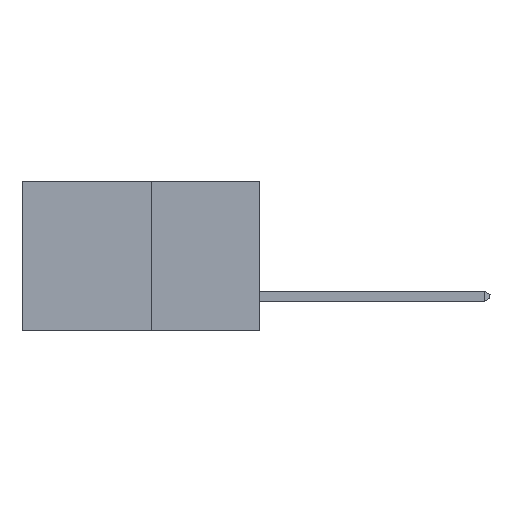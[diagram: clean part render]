
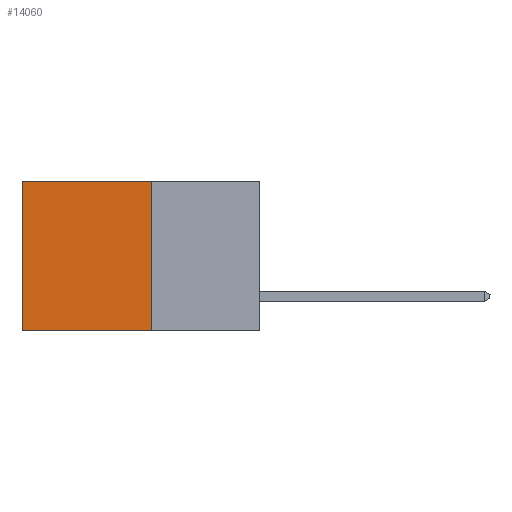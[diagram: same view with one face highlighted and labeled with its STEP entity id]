
A CAD part, left-side view. The second image highlights one B-rep face of the part: STEP entity #14060.
In plain terms, the highlighted planar face has unit normal (-1, 0, 0).
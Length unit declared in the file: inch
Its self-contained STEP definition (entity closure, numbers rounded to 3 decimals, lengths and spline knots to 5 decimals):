
#373 = CARTESIAN_POINT ( 'NONE',  ( 0.277, 0.59, -0.37 ) ) ;
#1002 = PLANE ( 'NONE',  #4621 ) ;
#1065 = EDGE_CURVE ( 'NONE', #9850, #3376, #4138, .T. ) ;
#1388 = VECTOR ( 'NONE', #14467, 39.37008 ) ;
#1573 = DIRECTION ( 'NONE',  ( 0., 0., -1. ) ) ;
#2392 = EDGE_LOOP ( 'NONE', ( #8125, #9862, #10087, #10769 ) ) ;
#2715 = CARTESIAN_POINT ( 'NONE',  ( 0.277, 0.27, -0.37 ) ) ;
#3339 = VECTOR ( 'NONE', #8155, 39.37008 ) ;
#3376 = VERTEX_POINT ( 'NONE', #4546 ) ;
#4138 = LINE ( 'NONE', #4902, #9516 ) ;
#4175 = LINE ( 'NONE', #6964, #1388 ) ;
#4546 = CARTESIAN_POINT ( 'NONE',  ( 0.277, 0.59, -0.37 ) ) ;
#4586 = DIRECTION ( 'NONE',  ( 1., 0., 0. ) ) ;
#4621 = AXIS2_PLACEMENT_3D ( 'NONE', #5686, #4586, #12361 ) ;
#4902 = CARTESIAN_POINT ( 'NONE',  ( 0.277, 0.27, -0.37 ) ) ;
#5686 = CARTESIAN_POINT ( 'NONE',  ( 0.277, 0.27, -0.37 ) ) ;
#5804 = CARTESIAN_POINT ( 'NONE',  ( 0.277, 0.59, 0. ) ) ;
#6320 = LINE ( 'NONE', #373, #9744 ) ;
#6578 = DIRECTION ( 'NONE',  ( 0., 1., 0. ) ) ;
#6732 = CARTESIAN_POINT ( 'NONE',  ( 0.277, 0.27, 0. ) ) ;
#6964 = CARTESIAN_POINT ( 'NONE',  ( 0.277, 0.27, -0.37 ) ) ;
#7525 = EDGE_CURVE ( 'NONE', #10479, #10148, #12274, .T. ) ;
#8125 = ORIENTED_EDGE ( 'NONE', *, *, #14337, .T. ) ;
#8155 = DIRECTION ( 'NONE',  ( 0., 1., 0. ) ) ;
#8643 = CARTESIAN_POINT ( 'NONE',  ( 0.277, 0.27, 0. ) ) ;
#9516 = VECTOR ( 'NONE', #6578, 39.37008 ) ;
#9744 = VECTOR ( 'NONE', #1573, 39.37008 ) ;
#9850 = VERTEX_POINT ( 'NONE', #2715 ) ;
#9862 = ORIENTED_EDGE ( 'NONE', *, *, #1065, .F. ) ;
#10087 = ORIENTED_EDGE ( 'NONE', *, *, #10161, .F. ) ;
#10148 = VERTEX_POINT ( 'NONE', #5804 ) ;
#10161 = EDGE_CURVE ( 'NONE', #10479, #9850, #4175, .T. ) ;
#10479 = VERTEX_POINT ( 'NONE', #8643 ) ;
#10769 = ORIENTED_EDGE ( 'NONE', *, *, #7525, .T. ) ;
#12274 = LINE ( 'NONE', #6732, #3339 ) ;
#12361 = DIRECTION ( 'NONE',  ( 0., 0., -1. ) ) ;
#13030 = FACE_OUTER_BOUND ( 'NONE', #2392, .T. ) ;
#14060 = ADVANCED_FACE ( 'NONE', ( #13030 ), #1002, .F. ) ;
#14337 = EDGE_CURVE ( 'NONE', #10148, #3376, #6320, .T. ) ;
#14467 = DIRECTION ( 'NONE',  ( 0., 0., -1. ) ) ;
